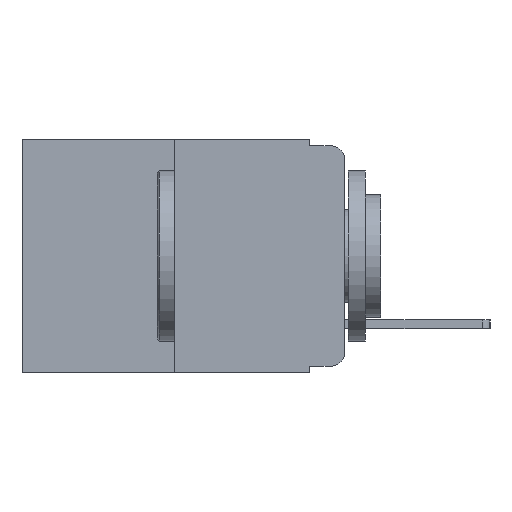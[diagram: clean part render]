
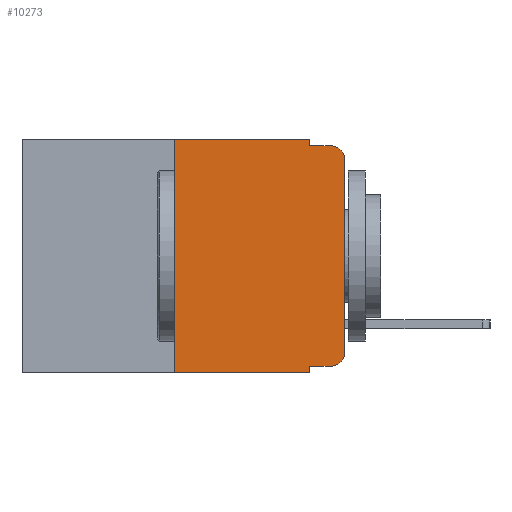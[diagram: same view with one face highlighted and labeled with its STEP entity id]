
A CAD part, left-side view. The second image highlights one B-rep face of the part: STEP entity #10273.
In plain terms, the highlighted planar face has unit normal (-1, 0, 0).
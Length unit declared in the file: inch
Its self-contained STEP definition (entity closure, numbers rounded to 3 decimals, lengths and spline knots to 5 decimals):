
#639 = CARTESIAN_POINT ( 'NONE',  ( 0., 0., -0.313 ) ) ;
#908 = PLANE ( 'NONE',  #13190 ) ;
#1281 = LINE ( 'NONE', #5934, #17424 ) ;
#1316 = FACE_OUTER_BOUND ( 'NONE', #12460, .T. ) ;
#1599 = EDGE_CURVE ( 'NONE', #19301, #4335, #1281, .T. ) ;
#1647 = CARTESIAN_POINT ( 'NONE',  ( 0., 0., 0. ) ) ;
#1678 = LINE ( 'NONE', #16375, #13730 ) ;
#1708 = VERTEX_POINT ( 'NONE', #11220 ) ;
#1929 = CARTESIAN_POINT ( 'NONE',  ( 0., 0.051, -0.01 ) ) ;
#1997 = LINE ( 'NONE', #2411, #5918 ) ;
#2357 = VECTOR ( 'NONE', #20416, 39.37008 ) ;
#2411 = CARTESIAN_POINT ( 'NONE',  ( 0., 0.051, -0.01 ) ) ;
#2421 = VERTEX_POINT ( 'NONE', #16862 ) ;
#2523 = ORIENTED_EDGE ( 'NONE', *, *, #1599, .F. ) ;
#2598 = DIRECTION ( 'NONE',  ( 1., 0., 0. ) ) ;
#2774 = ORIENTED_EDGE ( 'NONE', *, *, #20516, .T. ) ;
#3038 = LINE ( 'NONE', #1647, #6930 ) ;
#3442 = VERTEX_POINT ( 'NONE', #10035 ) ;
#4117 = DIRECTION ( 'NONE',  ( 0., -1., 0. ) ) ;
#4234 = ORIENTED_EDGE ( 'NONE', *, *, #13452, .F. ) ;
#4289 = EDGE_CURVE ( 'NONE', #19829, #19566, #1678, .T. ) ;
#4335 = VERTEX_POINT ( 'NONE', #1929 ) ;
#4418 = CARTESIAN_POINT ( 'NONE',  ( 0., 0.051, -0.343 ) ) ;
#4492 = CARTESIAN_POINT ( 'NONE',  ( 0., 0.02, -0.01 ) ) ;
#5107 = DIRECTION ( 'NONE',  ( 0., 0., 1. ) ) ;
#5271 = DIRECTION ( 'NONE',  ( -1., 0., 0. ) ) ;
#5403 = EDGE_CURVE ( 'NONE', #2421, #6107, #13923, .T. ) ;
#5918 = VECTOR ( 'NONE', #4117, 39.37008 ) ;
#5934 = CARTESIAN_POINT ( 'NONE',  ( 0., 0.051, 0. ) ) ;
#5990 = DIRECTION ( 'NONE',  ( 0., 0., -1. ) ) ;
#6107 = VERTEX_POINT ( 'NONE', #639 ) ;
#6575 = CARTESIAN_POINT ( 'NONE',  ( 0., 0.473, -0.343 ) ) ;
#6685 = ORIENTED_EDGE ( 'NONE', *, *, #8495, .T. ) ;
#6760 = DIRECTION ( 'NONE',  ( -1., 0., 0. ) ) ;
#6831 = LINE ( 'NONE', #6575, #10069 ) ;
#6930 = VECTOR ( 'NONE', #5107, 39.37008 ) ;
#8269 = DIRECTION ( 'NONE',  ( 0., 0., -1. ) ) ;
#8495 = EDGE_CURVE ( 'NONE', #3442, #19566, #6831, .T. ) ;
#8632 = ORIENTED_EDGE ( 'NONE', *, *, #18640, .T. ) ;
#8721 = VECTOR ( 'NONE', #12687, 39.37008 ) ;
#9029 = CARTESIAN_POINT ( 'NONE',  ( 0., 0.473, 0. ) ) ;
#9223 = LINE ( 'NONE', #11053, #8721 ) ;
#9903 = CARTESIAN_POINT ( 'NONE',  ( 0., 0.051, -0.333 ) ) ;
#9920 = CARTESIAN_POINT ( 'NONE',  ( 0., 0.051, 0. ) ) ;
#10035 = CARTESIAN_POINT ( 'NONE',  ( 0., 0.25, -0.343 ) ) ;
#10069 = VECTOR ( 'NONE', #13080, 39.37008 ) ;
#10273 = ADVANCED_FACE ( 'NONE', ( #1316 ), #908, .F. ) ;
#10883 = CARTESIAN_POINT ( 'NONE',  ( 0., 0., -0.03 ) ) ;
#11053 = CARTESIAN_POINT ( 'NONE',  ( 0., 0.473, 0. ) ) ;
#11220 = CARTESIAN_POINT ( 'NONE',  ( 0., 0.25, 0. ) ) ;
#12160 = LINE ( 'NONE', #16050, #15844 ) ;
#12460 = EDGE_LOOP ( 'NONE', ( #8632, #20282, #15096, #2523, #4234, #13707, #6685, #19899, #2774, #15860 ) ) ;
#12687 = DIRECTION ( 'NONE',  ( 0., -1., 0. ) ) ;
#12981 = AXIS2_PLACEMENT_3D ( 'NONE', #14928, #5271, #16463 ) ;
#13080 = DIRECTION ( 'NONE',  ( 0., -1., 0. ) ) ;
#13190 = AXIS2_PLACEMENT_3D ( 'NONE', #9029, #2598, #14008 ) ;
#13452 = EDGE_CURVE ( 'NONE', #1708, #19301, #9223, .T. ) ;
#13523 = EDGE_CURVE ( 'NONE', #14705, #19619, #20214, .T. ) ;
#13707 = ORIENTED_EDGE ( 'NONE', *, *, #16523, .F. ) ;
#13730 = VECTOR ( 'NONE', #8269, 39.37008 ) ;
#13923 = CIRCLE ( 'NONE', #12981, 0.02 ) ;
#14008 = DIRECTION ( 'NONE',  ( 0., 0., -1. ) ) ;
#14705 = VERTEX_POINT ( 'NONE', #10883 ) ;
#14928 = CARTESIAN_POINT ( 'NONE',  ( 0., 0.02, -0.313 ) ) ;
#15096 = ORIENTED_EDGE ( 'NONE', *, *, #18269, .F. ) ;
#15844 = VECTOR ( 'NONE', #20499, 39.37008 ) ;
#15860 = ORIENTED_EDGE ( 'NONE', *, *, #5403, .T. ) ;
#16009 = AXIS2_PLACEMENT_3D ( 'NONE', #16052, #6760, #17844 ) ;
#16050 = CARTESIAN_POINT ( 'NONE',  ( 0., 0.051, -0.333 ) ) ;
#16052 = CARTESIAN_POINT ( 'NONE',  ( 0., 0.02, -0.03 ) ) ;
#16375 = CARTESIAN_POINT ( 'NONE',  ( 0., 0.051, 0. ) ) ;
#16463 = DIRECTION ( 'NONE',  ( 0., 0., -1. ) ) ;
#16523 = EDGE_CURVE ( 'NONE', #3442, #1708, #19790, .T. ) ;
#16862 = CARTESIAN_POINT ( 'NONE',  ( 0., 0.02, -0.333 ) ) ;
#17424 = VECTOR ( 'NONE', #5990, 39.37008 ) ;
#17844 = DIRECTION ( 'NONE',  ( 0., 0., -1. ) ) ;
#18269 = EDGE_CURVE ( 'NONE', #4335, #19619, #1997, .T. ) ;
#18640 = EDGE_CURVE ( 'NONE', #6107, #14705, #3038, .T. ) ;
#18912 = CARTESIAN_POINT ( 'NONE',  ( 0., 0.25, 0. ) ) ;
#19301 = VERTEX_POINT ( 'NONE', #9920 ) ;
#19566 = VERTEX_POINT ( 'NONE', #4418 ) ;
#19619 = VERTEX_POINT ( 'NONE', #4492 ) ;
#19790 = LINE ( 'NONE', #18912, #2357 ) ;
#19829 = VERTEX_POINT ( 'NONE', #9903 ) ;
#19899 = ORIENTED_EDGE ( 'NONE', *, *, #4289, .F. ) ;
#20214 = CIRCLE ( 'NONE', #16009, 0.02 ) ;
#20282 = ORIENTED_EDGE ( 'NONE', *, *, #13523, .T. ) ;
#20416 = DIRECTION ( 'NONE',  ( 0., 0., 1. ) ) ;
#20499 = DIRECTION ( 'NONE',  ( 0., -1., 0. ) ) ;
#20516 = EDGE_CURVE ( 'NONE', #19829, #2421, #12160, .T. ) ;
